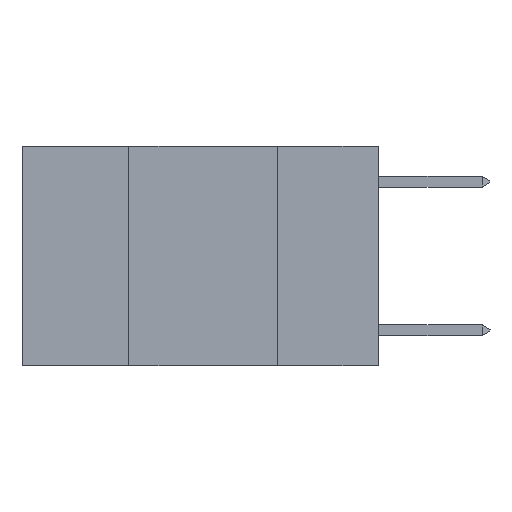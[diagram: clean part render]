
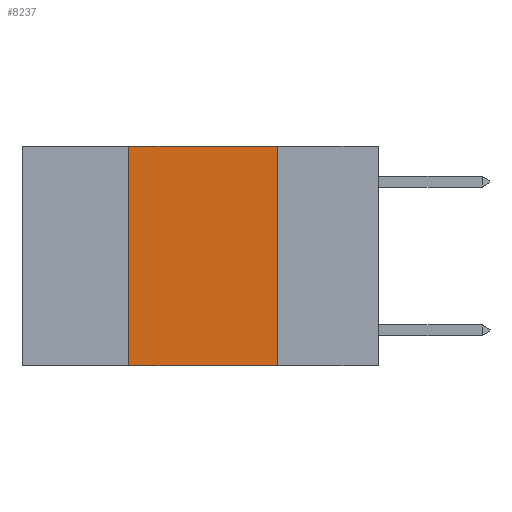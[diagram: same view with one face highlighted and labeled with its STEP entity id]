
A CAD part, left-side view. The second image highlights one B-rep face of the part: STEP entity #8237.
In plain terms, the highlighted planar face has unit normal (-1, 0, 0).
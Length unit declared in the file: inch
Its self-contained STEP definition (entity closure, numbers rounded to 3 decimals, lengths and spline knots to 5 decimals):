
#77 = VERTEX_POINT ( 'NONE', #8510 ) ;
#672 = CARTESIAN_POINT ( 'NONE',  ( 0., 0.42, -0.37 ) ) ;
#1936 = EDGE_LOOP ( 'NONE', ( #13204, #2188, #15391, #6432 ) ) ;
#2095 = VECTOR ( 'NONE', #12155, 39.37008 ) ;
#2188 = ORIENTED_EDGE ( 'NONE', *, *, #13437, .F. ) ;
#2615 = VERTEX_POINT ( 'NONE', #4411 ) ;
#3038 = CARTESIAN_POINT ( 'NONE',  ( 0., 0.6, 0. ) ) ;
#3076 = VERTEX_POINT ( 'NONE', #11378 ) ;
#3108 = DIRECTION ( 'NONE',  ( 0., -1., 0. ) ) ;
#3118 = FACE_OUTER_BOUND ( 'NONE', #1936, .T. ) ;
#3235 = EDGE_CURVE ( 'NONE', #12169, #2615, #12512, .T. ) ;
#3538 = CARTESIAN_POINT ( 'NONE',  ( 0., 0.42, 0. ) ) ;
#3782 = CARTESIAN_POINT ( 'NONE',  ( 0., 0.17, 0. ) ) ;
#4411 = CARTESIAN_POINT ( 'NONE',  ( 0., 0.17, -0.37 ) ) ;
#4428 = CARTESIAN_POINT ( 'NONE',  ( 0., 0.6, 0. ) ) ;
#5301 = AXIS2_PLACEMENT_3D ( 'NONE', #3038, #13987, #6818 ) ;
#5586 = PLANE ( 'NONE',  #5301 ) ;
#6229 = LINE ( 'NONE', #3782, #9068 ) ;
#6432 = ORIENTED_EDGE ( 'NONE', *, *, #3235, .T. ) ;
#6818 = DIRECTION ( 'NONE',  ( 0., 0., -1. ) ) ;
#8237 = ADVANCED_FACE ( 'NONE', ( #3118 ), #5586, .F. ) ;
#8510 = CARTESIAN_POINT ( 'NONE',  ( 0., 0.42, 0. ) ) ;
#8535 = EDGE_CURVE ( 'NONE', #12169, #77, #12305, .T. ) ;
#9068 = VECTOR ( 'NONE', #13552, 39.37008 ) ;
#9323 = VECTOR ( 'NONE', #3108, 39.37008 ) ;
#11378 = CARTESIAN_POINT ( 'NONE',  ( 0., 0.17, 0. ) ) ;
#11482 = LINE ( 'NONE', #4428, #14240 ) ;
#12155 = DIRECTION ( 'NONE',  ( 0., 0., 1. ) ) ;
#12169 = VERTEX_POINT ( 'NONE', #672 ) ;
#12305 = LINE ( 'NONE', #3538, #2095 ) ;
#12512 = LINE ( 'NONE', #15124, #9323 ) ;
#12554 = EDGE_CURVE ( 'NONE', #3076, #2615, #6229, .T. ) ;
#13204 = ORIENTED_EDGE ( 'NONE', *, *, #12554, .F. ) ;
#13437 = EDGE_CURVE ( 'NONE', #77, #3076, #11482, .T. ) ;
#13552 = DIRECTION ( 'NONE',  ( 0., 0., -1. ) ) ;
#13987 = DIRECTION ( 'NONE',  ( 1., 0., 0. ) ) ;
#14081 = DIRECTION ( 'NONE',  ( 0., -1., 0. ) ) ;
#14240 = VECTOR ( 'NONE', #14081, 39.37008 ) ;
#15124 = CARTESIAN_POINT ( 'NONE',  ( 0., 0.6, -0.37 ) ) ;
#15391 = ORIENTED_EDGE ( 'NONE', *, *, #8535, .F. ) ;
